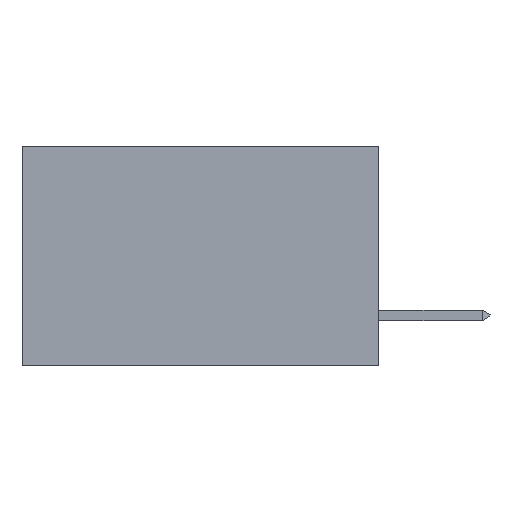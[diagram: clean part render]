
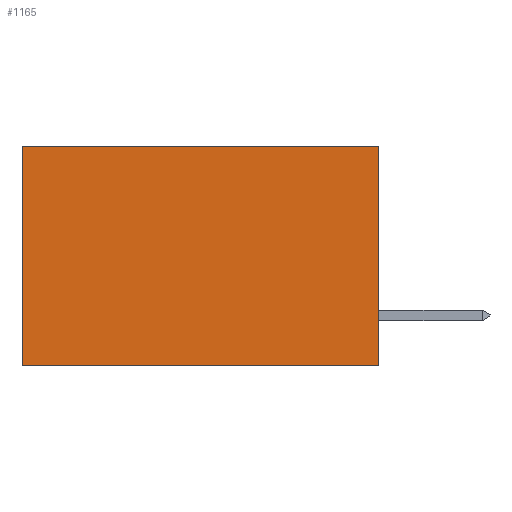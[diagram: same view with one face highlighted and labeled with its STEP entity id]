
A CAD part, left-side view. The second image highlights one B-rep face of the part: STEP entity #1165.
In plain terms, the highlighted planar face has unit normal (-1, 0, 0).
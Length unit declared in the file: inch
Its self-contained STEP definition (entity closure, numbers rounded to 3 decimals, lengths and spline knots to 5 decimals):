
#90 = DIRECTION ( 'NONE',  ( 0., 1., 0. ) ) ;
#407 = CARTESIAN_POINT ( 'NONE',  ( 0.2615, 0., 0. ) ) ;
#627 = CARTESIAN_POINT ( 'NONE',  ( 0.2615, 0., -0.37 ) ) ;
#667 = VECTOR ( 'NONE', #19704, 39.37008 ) ;
#1165 = ADVANCED_FACE ( 'NONE', ( #10100 ), #3337, .F. ) ;
#1365 = VERTEX_POINT ( 'NONE', #12024 ) ;
#1589 = VECTOR ( 'NONE', #3900, 39.37008 ) ;
#3337 = PLANE ( 'NONE',  #19287 ) ;
#3645 = LINE ( 'NONE', #6752, #667 ) ;
#3900 = DIRECTION ( 'NONE',  ( 0., 0., -1. ) ) ;
#4329 = EDGE_CURVE ( 'NONE', #19681, #1365, #9899, .T. ) ;
#5372 = EDGE_LOOP ( 'NONE', ( #13889, #21155, #20927, #11041 ) ) ;
#6752 = CARTESIAN_POINT ( 'NONE',  ( 0.2615, 0., 0. ) ) ;
#9899 = LINE ( 'NONE', #11491, #11483 ) ;
#10100 = FACE_OUTER_BOUND ( 'NONE', #5372, .T. ) ;
#10189 = CARTESIAN_POINT ( 'NONE',  ( 0.2615, 0.6, -0.37 ) ) ;
#11041 = ORIENTED_EDGE ( 'NONE', *, *, #18591, .T. ) ;
#11189 = EDGE_CURVE ( 'NONE', #12133, #19681, #19956, .T. ) ;
#11483 = VECTOR ( 'NONE', #90, 39.37008 ) ;
#11491 = CARTESIAN_POINT ( 'NONE',  ( 0.2615, 0., -0.37 ) ) ;
#11589 = DIRECTION ( 'NONE',  ( 0., 0., -1. ) ) ;
#11825 = CARTESIAN_POINT ( 'NONE',  ( 0.2615, 0., -0.37 ) ) ;
#12024 = CARTESIAN_POINT ( 'NONE',  ( 0.2615, 0.6, -0.37 ) ) ;
#12133 = VERTEX_POINT ( 'NONE', #407 ) ;
#12144 = EDGE_CURVE ( 'NONE', #12389, #1365, #20339, .T. ) ;
#12389 = VERTEX_POINT ( 'NONE', #15156 ) ;
#12868 = VECTOR ( 'NONE', #13596, 39.37008 ) ;
#13596 = DIRECTION ( 'NONE',  ( 0., 0., -1. ) ) ;
#13889 = ORIENTED_EDGE ( 'NONE', *, *, #12144, .T. ) ;
#14900 = CARTESIAN_POINT ( 'NONE',  ( 0.2615, 0., -0.37 ) ) ;
#15156 = CARTESIAN_POINT ( 'NONE',  ( 0.2615, 0.6, 0. ) ) ;
#18591 = EDGE_CURVE ( 'NONE', #12133, #12389, #3645, .T. ) ;
#19287 = AXIS2_PLACEMENT_3D ( 'NONE', #14900, #19712, #11589 ) ;
#19681 = VERTEX_POINT ( 'NONE', #627 ) ;
#19704 = DIRECTION ( 'NONE',  ( 0., 1., 0. ) ) ;
#19712 = DIRECTION ( 'NONE',  ( 1., 0., 0. ) ) ;
#19956 = LINE ( 'NONE', #11825, #1589 ) ;
#20339 = LINE ( 'NONE', #10189, #12868 ) ;
#20927 = ORIENTED_EDGE ( 'NONE', *, *, #11189, .F. ) ;
#21155 = ORIENTED_EDGE ( 'NONE', *, *, #4329, .F. ) ;
